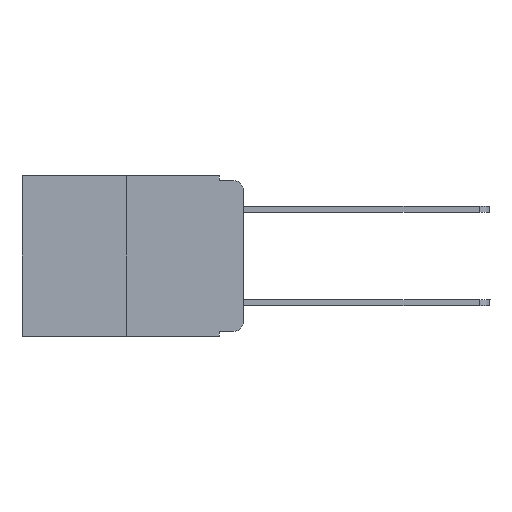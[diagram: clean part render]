
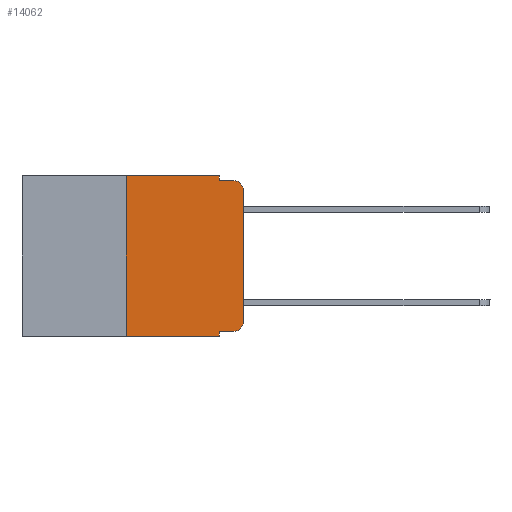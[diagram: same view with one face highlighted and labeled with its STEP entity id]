
A CAD part, left-side view. The second image highlights one B-rep face of the part: STEP entity #14062.
In plain terms, the highlighted planar face has unit normal (-1, 0, 0).
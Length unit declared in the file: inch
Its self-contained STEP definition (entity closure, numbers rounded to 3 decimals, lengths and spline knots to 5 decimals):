
#82 = CARTESIAN_POINT ( 'NONE',  ( 0., 0.051, -0.333 ) ) ;
#294 = LINE ( 'NONE', #4859, #3589 ) ;
#349 = EDGE_CURVE ( 'NONE', #551, #409, #11153, .T. ) ;
#409 = VERTEX_POINT ( 'NONE', #2082 ) ;
#460 = VERTEX_POINT ( 'NONE', #13837 ) ;
#551 = VERTEX_POINT ( 'NONE', #13013 ) ;
#563 = VECTOR ( 'NONE', #13620, 39.37008 ) ;
#738 = VERTEX_POINT ( 'NONE', #5105 ) ;
#745 = DIRECTION ( 'NONE',  ( 0., 0., 1. ) ) ;
#989 = CARTESIAN_POINT ( 'NONE',  ( 0., 0., -0.03 ) ) ;
#1064 = CARTESIAN_POINT ( 'NONE',  ( 0., 0.473, 0. ) ) ;
#1207 = CARTESIAN_POINT ( 'NONE',  ( 0., 0.051, -0.01 ) ) ;
#1219 = DIRECTION ( 'NONE',  ( 0., 0., -1. ) ) ;
#1380 = VECTOR ( 'NONE', #8600, 39.37008 ) ;
#1508 = CARTESIAN_POINT ( 'NONE',  ( 0., 0.02, -0.01 ) ) ;
#2082 = CARTESIAN_POINT ( 'NONE',  ( 0., 0.25, 0. ) ) ;
#2245 = DIRECTION ( 'NONE',  ( 0., 0., -1. ) ) ;
#2992 = DIRECTION ( 'NONE',  ( 0., 0., -1. ) ) ;
#3138 = CIRCLE ( 'NONE', #11504, 0.02 ) ;
#3223 = ORIENTED_EDGE ( 'NONE', *, *, #7943, .F. ) ;
#3350 = VERTEX_POINT ( 'NONE', #7158 ) ;
#3589 = VECTOR ( 'NONE', #745, 39.37008 ) ;
#3818 = VECTOR ( 'NONE', #5332, 39.37008 ) ;
#4427 = CARTESIAN_POINT ( 'NONE',  ( 0., 0.02, -0.333 ) ) ;
#4439 = PLANE ( 'NONE',  #9417 ) ;
#4609 = VECTOR ( 'NONE', #1219, 39.37008 ) ;
#4733 = CARTESIAN_POINT ( 'NONE',  ( 0., 0.02, -0.313 ) ) ;
#4859 = CARTESIAN_POINT ( 'NONE',  ( 0., 0., 0. ) ) ;
#4906 = VERTEX_POINT ( 'NONE', #1508 ) ;
#5105 = CARTESIAN_POINT ( 'NONE',  ( 0., 0.051, -0.333 ) ) ;
#5184 = ORIENTED_EDGE ( 'NONE', *, *, #8061, .T. ) ;
#5252 = ORIENTED_EDGE ( 'NONE', *, *, #5494, .T. ) ;
#5332 = DIRECTION ( 'NONE',  ( 0., -1., 0. ) ) ;
#5454 = DIRECTION ( 'NONE',  ( 0., 0., 1. ) ) ;
#5494 = EDGE_CURVE ( 'NONE', #551, #12543, #14197, .T. ) ;
#5605 = DIRECTION ( 'NONE',  ( -1., 0., 0. ) ) ;
#5768 = EDGE_LOOP ( 'NONE', ( #11954, #14515, #10319, #7019, #3223, #7985, #5252, #7015, #14710, #5184 ) ) ;
#6127 = VECTOR ( 'NONE', #5454, 39.37008 ) ;
#6439 = CARTESIAN_POINT ( 'NONE',  ( 0., 0.02, -0.03 ) ) ;
#6689 = CARTESIAN_POINT ( 'NONE',  ( 0., 0.473, 0. ) ) ;
#6829 = DIRECTION ( 'NONE',  ( -1., 0., 0. ) ) ;
#7015 = ORIENTED_EDGE ( 'NONE', *, *, #14620, .F. ) ;
#7019 = ORIENTED_EDGE ( 'NONE', *, *, #7314, .F. ) ;
#7158 = CARTESIAN_POINT ( 'NONE',  ( 0., 0., -0.313 ) ) ;
#7224 = CARTESIAN_POINT ( 'NONE',  ( 0., 0.051, -0.343 ) ) ;
#7314 = EDGE_CURVE ( 'NONE', #11306, #460, #14253, .T. ) ;
#7402 = CARTESIAN_POINT ( 'NONE',  ( 0., 0.473, -0.343 ) ) ;
#7600 = DIRECTION ( 'NONE',  ( 1., 0., 0. ) ) ;
#7903 = VERTEX_POINT ( 'NONE', #4427 ) ;
#7943 = EDGE_CURVE ( 'NONE', #409, #11306, #13551, .T. ) ;
#7985 = ORIENTED_EDGE ( 'NONE', *, *, #349, .F. ) ;
#8061 = EDGE_CURVE ( 'NONE', #7903, #3350, #12184, .T. ) ;
#8600 = DIRECTION ( 'NONE',  ( 0., -1., 0. ) ) ;
#8607 = AXIS2_PLACEMENT_3D ( 'NONE', #4733, #6829, #2245 ) ;
#8761 = CARTESIAN_POINT ( 'NONE',  ( 0., 0.25, 0. ) ) ;
#9142 = LINE ( 'NONE', #82, #563 ) ;
#9417 = AXIS2_PLACEMENT_3D ( 'NONE', #6689, #7600, #12378 ) ;
#9634 = DIRECTION ( 'NONE',  ( 0., 0., -1. ) ) ;
#9689 = CARTESIAN_POINT ( 'NONE',  ( 0., 0.051, 0. ) ) ;
#10003 = VECTOR ( 'NONE', #9634, 39.37008 ) ;
#10073 = VECTOR ( 'NONE', #13608, 39.37008 ) ;
#10128 = FACE_OUTER_BOUND ( 'NONE', #5768, .T. ) ;
#10319 = ORIENTED_EDGE ( 'NONE', *, *, #12036, .F. ) ;
#10494 = EDGE_CURVE ( 'NONE', #3350, #14436, #294, .T. ) ;
#10693 = LINE ( 'NONE', #1207, #10073 ) ;
#11153 = LINE ( 'NONE', #8761, #6127 ) ;
#11306 = VERTEX_POINT ( 'NONE', #9689 ) ;
#11312 = LINE ( 'NONE', #12437, #4609 ) ;
#11504 = AXIS2_PLACEMENT_3D ( 'NONE', #6439, #5605, #2992 ) ;
#11954 = ORIENTED_EDGE ( 'NONE', *, *, #10494, .T. ) ;
#11976 = EDGE_CURVE ( 'NONE', #14436, #4906, #3138, .T. ) ;
#12036 = EDGE_CURVE ( 'NONE', #460, #4906, #10693, .T. ) ;
#12184 = CIRCLE ( 'NONE', #8607, 0.02 ) ;
#12378 = DIRECTION ( 'NONE',  ( 0., 0., -1. ) ) ;
#12437 = CARTESIAN_POINT ( 'NONE',  ( 0., 0.051, 0. ) ) ;
#12543 = VERTEX_POINT ( 'NONE', #7224 ) ;
#13013 = CARTESIAN_POINT ( 'NONE',  ( 0., 0.25, -0.343 ) ) ;
#13073 = CARTESIAN_POINT ( 'NONE',  ( 0., 0.051, 0. ) ) ;
#13551 = LINE ( 'NONE', #1064, #3818 ) ;
#13608 = DIRECTION ( 'NONE',  ( 0., -1., 0. ) ) ;
#13620 = DIRECTION ( 'NONE',  ( 0., -1., 0. ) ) ;
#13837 = CARTESIAN_POINT ( 'NONE',  ( 0., 0.051, -0.01 ) ) ;
#14062 = ADVANCED_FACE ( 'NONE', ( #10128 ), #4439, .F. ) ;
#14197 = LINE ( 'NONE', #7402, #1380 ) ;
#14253 = LINE ( 'NONE', #13073, #10003 ) ;
#14436 = VERTEX_POINT ( 'NONE', #989 ) ;
#14515 = ORIENTED_EDGE ( 'NONE', *, *, #11976, .T. ) ;
#14620 = EDGE_CURVE ( 'NONE', #738, #12543, #11312, .T. ) ;
#14635 = EDGE_CURVE ( 'NONE', #738, #7903, #9142, .T. ) ;
#14710 = ORIENTED_EDGE ( 'NONE', *, *, #14635, .T. ) ;
